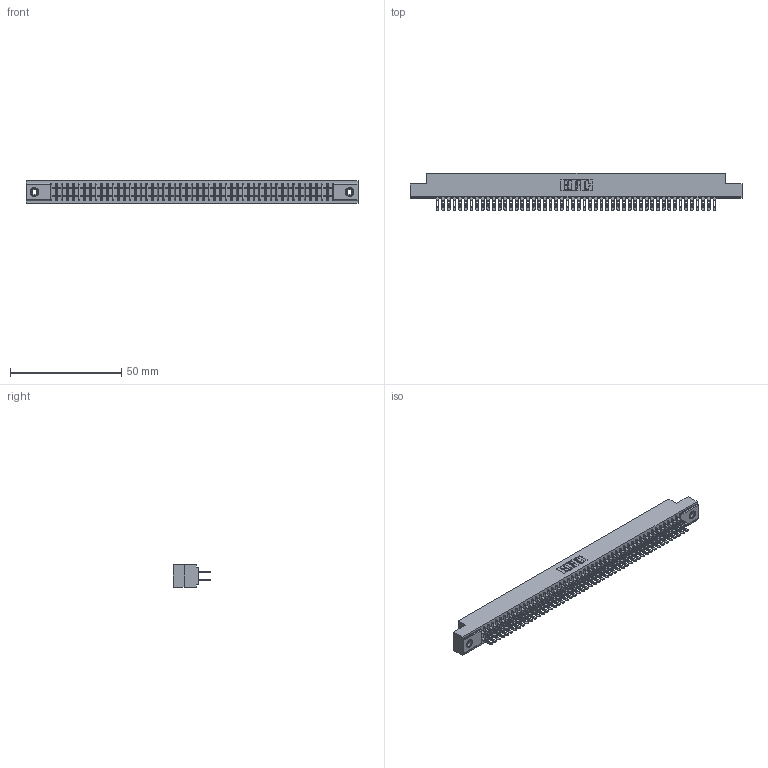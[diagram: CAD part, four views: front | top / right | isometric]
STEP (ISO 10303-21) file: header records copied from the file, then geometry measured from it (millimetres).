
FILE_DESCRIPTION (( 'STEP AP203' ), '1' );
FILE_NAME ('341-100-500-208.STEP', '2018-08-08T02:37:26', ( '' ), ( '' ), 'SwSTEP 2.0', 'SolidWorks 2016', '' );
FILE_SCHEMA (( 'CONFIG_CONTROL_DESIGN' ));
Products named in the file (4): 341 Part_.156 (3.96) Dia Mounting Holes; 341-292-001_341-292-100; 345-250-001_345-250-003-102; 341-100-500-208
Assembly tree (103 placements, depth 2):
  341-100-500-208
    341 Part_.156 (3.96) Dia Mounting Holes
    341-292-001_341-292-100  x100
    345-250-001_345-250-003-102  x2
Bounding box: 149.22 x 16.69 x 10.16 mm (x, y, z)
Volume: 11149.2 mm3; surface area: 20896.3 mm2
Topology: 103 solids, 103 shells, 6776 faces, 19602 edges, 12690 vertices
Faces by surface type: plane 3900, cylinder 2660, sphere 102, torus 102, cone 12
Entity records: 60638 total; most frequent: CARTESIAN_POINT 10061, ORIENTED_EDGE 9992, DIRECTION 9772, EDGE_CURVE 4996, VECTOR 4038, LINE 4038, VERTEX_POINT 3156, AXIS2_PLACEMENT_3D 2867
